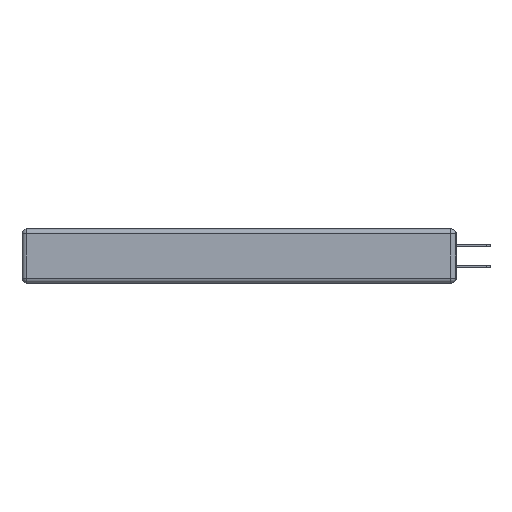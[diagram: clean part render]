
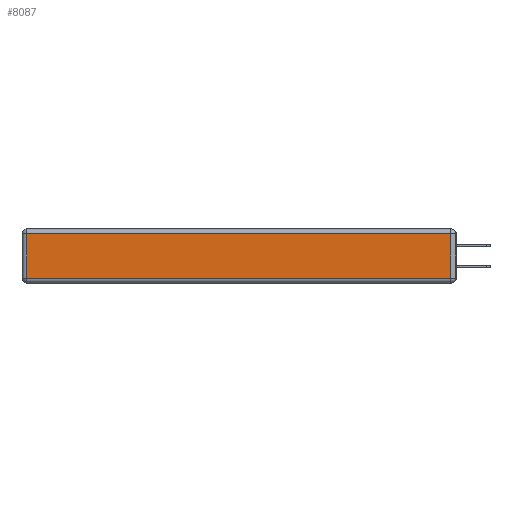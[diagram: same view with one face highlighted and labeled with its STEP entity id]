
A CAD part, left-side view. The second image highlights one B-rep face of the part: STEP entity #8087.
In plain terms, the highlighted planar face has unit normal (-1, 0, 0).
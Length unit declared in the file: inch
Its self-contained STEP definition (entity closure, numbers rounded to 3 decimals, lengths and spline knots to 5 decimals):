
#361 = VERTEX_POINT ( 'NONE', #10358 ) ;
#447 = DIRECTION ( 'NONE',  ( -1., 0., 0. ) ) ;
#1061 = ORIENTED_EDGE ( 'NONE', *, *, #12237, .T. ) ;
#1126 = CARTESIAN_POINT ( 'NONE',  ( 0., 2.75, -0.03 ) ) ;
#1170 = ORIENTED_EDGE ( 'NONE', *, *, #7826, .T. ) ;
#1294 = VECTOR ( 'NONE', #8536, 39.37008 ) ;
#1768 = DIRECTION ( 'NONE',  ( 0., -1., 0. ) ) ;
#2559 = DIRECTION ( 'NONE',  ( 0., 1., 0. ) ) ;
#2918 = EDGE_LOOP ( 'NONE', ( #1061, #1170, #14889, #15465 ) ) ;
#2956 = CARTESIAN_POINT ( 'NONE',  ( 0., 0., -0.343 ) ) ;
#3470 = VECTOR ( 'NONE', #2559, 39.37008 ) ;
#4348 = AXIS2_PLACEMENT_3D ( 'NONE', #2956, #447, #9315 ) ;
#4866 = CARTESIAN_POINT ( 'NONE',  ( 0., 2.72, -0.343 ) ) ;
#5086 = VERTEX_POINT ( 'NONE', #8368 ) ;
#5194 = PLANE ( 'NONE',  #4348 ) ;
#5859 = LINE ( 'NONE', #12279, #1294 ) ;
#6158 = EDGE_CURVE ( 'NONE', #7406, #361, #12864, .T. ) ;
#7406 = VERTEX_POINT ( 'NONE', #10053 ) ;
#7796 = LINE ( 'NONE', #7984, #9177 ) ;
#7826 = EDGE_CURVE ( 'NONE', #5086, #7406, #5859, .T. ) ;
#7984 = CARTESIAN_POINT ( 'NONE',  ( 0., 0., -0.313 ) ) ;
#8087 = ADVANCED_FACE ( 'NONE', ( #12622 ), #5194, .T. ) ;
#8215 = EDGE_CURVE ( 'NONE', #361, #12348, #15189, .T. ) ;
#8368 = CARTESIAN_POINT ( 'NONE',  ( 0., 0.03, -0.313 ) ) ;
#8536 = DIRECTION ( 'NONE',  ( 0., 0., 1. ) ) ;
#9177 = VECTOR ( 'NONE', #1768, 39.37008 ) ;
#9315 = DIRECTION ( 'NONE',  ( 0., 0., 1. ) ) ;
#9993 = DIRECTION ( 'NONE',  ( 0., 0., -1. ) ) ;
#10053 = CARTESIAN_POINT ( 'NONE',  ( 0., 0.03, -0.03 ) ) ;
#10358 = CARTESIAN_POINT ( 'NONE',  ( 0., 2.72, -0.03 ) ) ;
#12237 = EDGE_CURVE ( 'NONE', #12348, #5086, #7796, .T. ) ;
#12279 = CARTESIAN_POINT ( 'NONE',  ( 0., 0.03, -0.343 ) ) ;
#12348 = VERTEX_POINT ( 'NONE', #13410 ) ;
#12622 = FACE_OUTER_BOUND ( 'NONE', #2918, .T. ) ;
#12864 = LINE ( 'NONE', #1126, #3470 ) ;
#13410 = CARTESIAN_POINT ( 'NONE',  ( 0., 2.72, -0.313 ) ) ;
#13797 = VECTOR ( 'NONE', #9993, 39.37008 ) ;
#14889 = ORIENTED_EDGE ( 'NONE', *, *, #6158, .T. ) ;
#15189 = LINE ( 'NONE', #4866, #13797 ) ;
#15465 = ORIENTED_EDGE ( 'NONE', *, *, #8215, .T. ) ;
